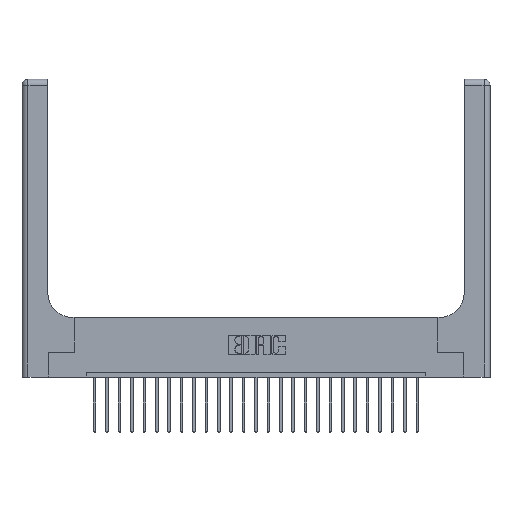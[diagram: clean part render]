
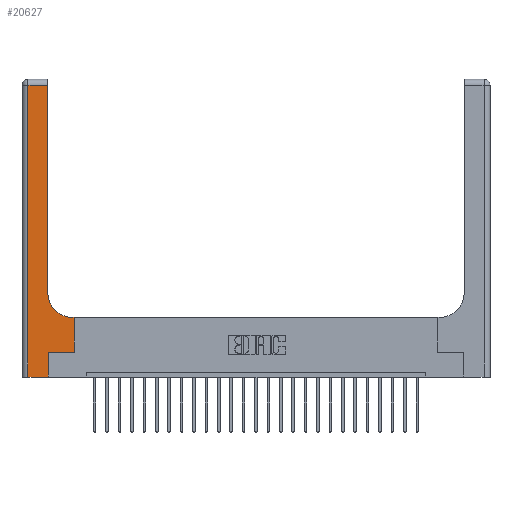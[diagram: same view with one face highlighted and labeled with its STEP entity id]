
A CAD part, top view. The second image highlights one B-rep face of the part: STEP entity #20627.
In plain terms, the highlighted planar face has unit normal (0, 0, 1).
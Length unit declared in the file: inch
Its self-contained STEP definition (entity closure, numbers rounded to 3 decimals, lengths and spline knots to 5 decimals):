
#239 = VERTEX_POINT ( 'NONE', #19208 ) ;
#678 = LINE ( 'NONE', #1550, #14906 ) ;
#816 = AXIS2_PLACEMENT_3D ( 'NONE', #18858, #20709, #15239 ) ;
#941 = VECTOR ( 'NONE', #3333, 39.37008 ) ;
#956 = DIRECTION ( 'NONE',  ( 0., 1., 0. ) ) ;
#1143 = LINE ( 'NONE', #6746, #4334 ) ;
#1335 = VERTEX_POINT ( 'NONE', #21386 ) ;
#1550 = CARTESIAN_POINT ( 'NONE',  ( 0.06, 3., 0.37 ) ) ;
#2483 = CARTESIAN_POINT ( 'NONE',  ( 0.06, 0., 0.37 ) ) ;
#2573 = CARTESIAN_POINT ( 'NONE',  ( 0.51, 0.6, 0.37 ) ) ;
#3120 = VECTOR ( 'NONE', #956, 39.37008 ) ;
#3333 = DIRECTION ( 'NONE',  ( -1., 0., 0. ) ) ;
#4334 = VECTOR ( 'NONE', #16029, 39.37008 ) ;
#4836 = CARTESIAN_POINT ( 'NONE',  ( 0.06, 2.94, 0.37 ) ) ;
#5453 = DIRECTION ( 'NONE',  ( 1., 0., 0. ) ) ;
#5711 = ORIENTED_EDGE ( 'NONE', *, *, #13646, .T. ) ;
#5778 = VERTEX_POINT ( 'NONE', #4836 ) ;
#5988 = VECTOR ( 'NONE', #15088, 39.37008 ) ;
#6534 = LINE ( 'NONE', #17837, #20792 ) ;
#6711 = DIRECTION ( 'NONE',  ( 0., 1., 0. ) ) ;
#6746 = CARTESIAN_POINT ( 'NONE',  ( 0.26, 0.6, 0.37 ) ) ;
#6754 = VECTOR ( 'NONE', #17710, 39.37008 ) ;
#6925 = EDGE_CURVE ( 'NONE', #239, #1335, #8115, .T. ) ;
#6983 = EDGE_CURVE ( 'NONE', #13435, #19822, #22047, .T. ) ;
#7336 = DIRECTION ( 'NONE',  ( 0., 0., -1. ) ) ;
#7815 = LINE ( 'NONE', #12132, #6754 ) ;
#7865 = EDGE_CURVE ( 'NONE', #13055, #5778, #16331, .T. ) ;
#8115 = LINE ( 'NONE', #15463, #3120 ) ;
#8641 = VERTEX_POINT ( 'NONE', #23299 ) ;
#9985 = ORIENTED_EDGE ( 'NONE', *, *, #6983, .T. ) ;
#11057 = ORIENTED_EDGE ( 'NONE', *, *, #19225, .T. ) ;
#11415 = EDGE_CURVE ( 'NONE', #17827, #239, #7815, .T. ) ;
#12005 = EDGE_CURVE ( 'NONE', #8641, #17827, #6534, .T. ) ;
#12132 = CARTESIAN_POINT ( 'NONE',  ( 0.265, 0.25, 0.37 ) ) ;
#12844 = VECTOR ( 'NONE', #18916, 39.37008 ) ;
#13055 = VERTEX_POINT ( 'NONE', #20248 ) ;
#13195 = CARTESIAN_POINT ( 'NONE',  ( 0., 0., 0.37 ) ) ;
#13435 = VERTEX_POINT ( 'NONE', #2573 ) ;
#13646 = EDGE_CURVE ( 'NONE', #5778, #19915, #678, .T. ) ;
#13762 = EDGE_CURVE ( 'NONE', #19822, #13055, #20558, .T. ) ;
#14309 = LINE ( 'NONE', #13195, #12844 ) ;
#14906 = VECTOR ( 'NONE', #23999, 39.37008 ) ;
#15088 = DIRECTION ( 'NONE',  ( 0., 1., 0. ) ) ;
#15239 = DIRECTION ( 'NONE',  ( -1., 0., 0. ) ) ;
#15463 = CARTESIAN_POINT ( 'NONE',  ( 0.528, 0.25, 0.37 ) ) ;
#16029 = DIRECTION ( 'NONE',  ( -1., 0., 0. ) ) ;
#16331 = LINE ( 'NONE', #21848, #941 ) ;
#16789 = CARTESIAN_POINT ( 'NONE',  ( 0.265, 0.25, 0.37 ) ) ;
#16828 = CARTESIAN_POINT ( 'NONE',  ( 0.26, 0.85, 0.37 ) ) ;
#16890 = CARTESIAN_POINT ( 'NONE',  ( 0.26, 3., 0.37 ) ) ;
#17044 = FACE_OUTER_BOUND ( 'NONE', #20090, .T. ) ;
#17710 = DIRECTION ( 'NONE',  ( 1., 0., 0. ) ) ;
#17743 = AXIS2_PLACEMENT_3D ( 'NONE', #22321, #7336, #5453 ) ;
#17827 = VERTEX_POINT ( 'NONE', #16789 ) ;
#17837 = CARTESIAN_POINT ( 'NONE',  ( 0.265, 0., 0.37 ) ) ;
#18171 = EDGE_CURVE ( 'NONE', #19915, #8641, #14309, .T. ) ;
#18858 = CARTESIAN_POINT ( 'NONE',  ( 0., 3., 0.37 ) ) ;
#18916 = DIRECTION ( 'NONE',  ( 1., 0., 0. ) ) ;
#19208 = CARTESIAN_POINT ( 'NONE',  ( 0.528, 0.25, 0.37 ) ) ;
#19225 = EDGE_CURVE ( 'NONE', #1335, #13435, #1143, .T. ) ;
#19822 = VERTEX_POINT ( 'NONE', #16828 ) ;
#19915 = VERTEX_POINT ( 'NONE', #2483 ) ;
#20090 = EDGE_LOOP ( 'NONE', ( #21342, #20500, #5711, #22194, #20278, #22186, #20620, #11057, #9985 ) ) ;
#20248 = CARTESIAN_POINT ( 'NONE',  ( 0.26, 2.94, 0.37 ) ) ;
#20278 = ORIENTED_EDGE ( 'NONE', *, *, #12005, .T. ) ;
#20500 = ORIENTED_EDGE ( 'NONE', *, *, #7865, .T. ) ;
#20558 = LINE ( 'NONE', #16890, #5988 ) ;
#20620 = ORIENTED_EDGE ( 'NONE', *, *, #6925, .T. ) ;
#20627 = ADVANCED_FACE ( 'NONE', ( #17044 ), #22529, .F. ) ;
#20709 = DIRECTION ( 'NONE',  ( 0., 0., -1. ) ) ;
#20792 = VECTOR ( 'NONE', #6711, 39.37008 ) ;
#21342 = ORIENTED_EDGE ( 'NONE', *, *, #13762, .T. ) ;
#21386 = CARTESIAN_POINT ( 'NONE',  ( 0.528, 0.6, 0.37 ) ) ;
#21848 = CARTESIAN_POINT ( 'NONE',  ( 0., 2.94, 0.37 ) ) ;
#22047 = CIRCLE ( 'NONE', #17743, 0.25 ) ;
#22186 = ORIENTED_EDGE ( 'NONE', *, *, #11415, .T. ) ;
#22194 = ORIENTED_EDGE ( 'NONE', *, *, #18171, .T. ) ;
#22321 = CARTESIAN_POINT ( 'NONE',  ( 0.51, 0.85, 0.37 ) ) ;
#22529 = PLANE ( 'NONE',  #816 ) ;
#23299 = CARTESIAN_POINT ( 'NONE',  ( 0.265, 0., 0.37 ) ) ;
#23999 = DIRECTION ( 'NONE',  ( 0., -1., 0. ) ) ;
